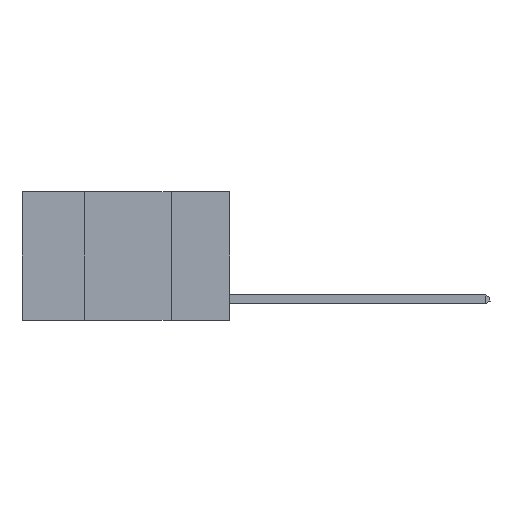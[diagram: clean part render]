
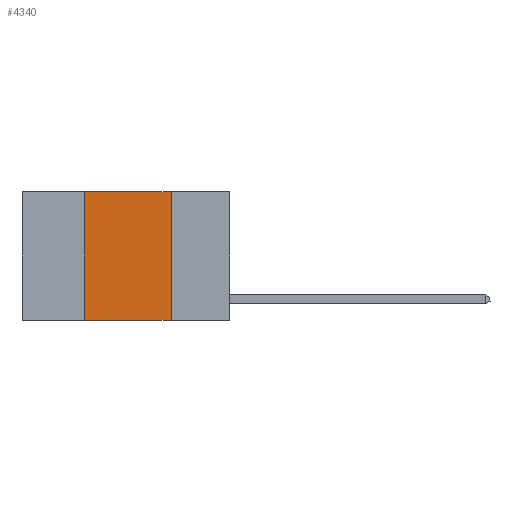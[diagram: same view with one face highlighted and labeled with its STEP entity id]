
A CAD part, left-side view. The second image highlights one B-rep face of the part: STEP entity #4340.
In plain terms, the highlighted planar face has unit normal (-1, 0, 0).
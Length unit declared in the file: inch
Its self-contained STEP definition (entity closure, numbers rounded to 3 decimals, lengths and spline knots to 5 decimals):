
#45 = DIRECTION ( 'NONE',  ( 0., 0., 1. ) ) ;
#388 = ORIENTED_EDGE ( 'NONE', *, *, #11115, .F. ) ;
#425 = VECTOR ( 'NONE', #10952, 39.37008 ) ;
#1078 = LINE ( 'NONE', #12052, #425 ) ;
#1166 = LINE ( 'NONE', #5025, #11690 ) ;
#1593 = ORIENTED_EDGE ( 'NONE', *, *, #7993, .T. ) ;
#1699 = ORIENTED_EDGE ( 'NONE', *, *, #11702, .F. ) ;
#2251 = CARTESIAN_POINT ( 'NONE',  ( 0., 0.42, -0.37 ) ) ;
#2331 = VERTEX_POINT ( 'NONE', #7932 ) ;
#2357 = VERTEX_POINT ( 'NONE', #7701 ) ;
#2638 = CARTESIAN_POINT ( 'NONE',  ( 0., 0.6, 0. ) ) ;
#3278 = CARTESIAN_POINT ( 'NONE',  ( 0., 0.42, 0. ) ) ;
#3348 = LINE ( 'NONE', #3278, #7559 ) ;
#4340 = ADVANCED_FACE ( 'NONE', ( #4857 ), #11891, .F. ) ;
#4645 = DIRECTION ( 'NONE',  ( 0., 0., -1. ) ) ;
#4857 = FACE_OUTER_BOUND ( 'NONE', #13252, .T. ) ;
#5025 = CARTESIAN_POINT ( 'NONE',  ( 0., 0.17, 0. ) ) ;
#7559 = VECTOR ( 'NONE', #45, 39.37008 ) ;
#7701 = CARTESIAN_POINT ( 'NONE',  ( 0., 0.17, 0. ) ) ;
#7932 = CARTESIAN_POINT ( 'NONE',  ( 0., 0.17, -0.37 ) ) ;
#7993 = EDGE_CURVE ( 'NONE', #10954, #2331, #1078, .T. ) ;
#8565 = CARTESIAN_POINT ( 'NONE',  ( 0., 0.6, 0. ) ) ;
#9760 = EDGE_CURVE ( 'NONE', #11427, #2357, #12208, .T. ) ;
#9857 = DIRECTION ( 'NONE',  ( 1., 0., 0. ) ) ;
#10168 = CARTESIAN_POINT ( 'NONE',  ( 0., 0.42, 0. ) ) ;
#10569 = VECTOR ( 'NONE', #11559, 39.37008 ) ;
#10874 = AXIS2_PLACEMENT_3D ( 'NONE', #2638, #9857, #4645 ) ;
#10952 = DIRECTION ( 'NONE',  ( 0., -1., 0. ) ) ;
#10954 = VERTEX_POINT ( 'NONE', #2251 ) ;
#11115 = EDGE_CURVE ( 'NONE', #10954, #11427, #3348, .T. ) ;
#11427 = VERTEX_POINT ( 'NONE', #10168 ) ;
#11559 = DIRECTION ( 'NONE',  ( 0., -1., 0. ) ) ;
#11637 = ORIENTED_EDGE ( 'NONE', *, *, #9760, .F. ) ;
#11690 = VECTOR ( 'NONE', #12759, 39.37008 ) ;
#11702 = EDGE_CURVE ( 'NONE', #2357, #2331, #1166, .T. ) ;
#11891 = PLANE ( 'NONE',  #10874 ) ;
#12052 = CARTESIAN_POINT ( 'NONE',  ( 0., 0.6, -0.37 ) ) ;
#12208 = LINE ( 'NONE', #8565, #10569 ) ;
#12759 = DIRECTION ( 'NONE',  ( 0., 0., -1. ) ) ;
#13252 = EDGE_LOOP ( 'NONE', ( #1699, #11637, #388, #1593 ) ) ;
